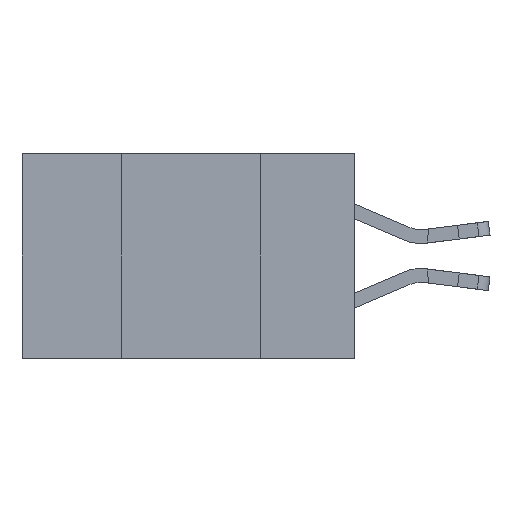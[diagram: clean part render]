
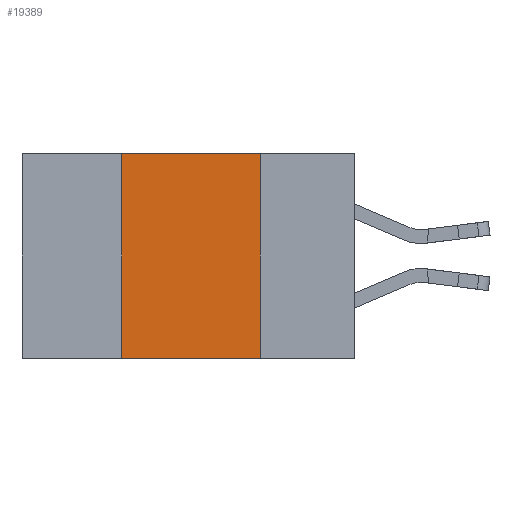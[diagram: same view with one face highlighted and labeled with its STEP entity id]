
A CAD part, left-side view. The second image highlights one B-rep face of the part: STEP entity #19389.
In plain terms, the highlighted planar face has unit normal (-1, 0, 0).
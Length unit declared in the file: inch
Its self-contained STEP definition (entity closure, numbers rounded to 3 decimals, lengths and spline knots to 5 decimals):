
#376 = VERTEX_POINT ( 'NONE', #18928 ) ;
#481 = DIRECTION ( 'NONE',  ( 0., 0., -1. ) ) ;
#744 = DIRECTION ( 'NONE',  ( 1., 0., 0. ) ) ;
#2223 = CARTESIAN_POINT ( 'NONE',  ( 0., 0.6, -0.37 ) ) ;
#2421 = VECTOR ( 'NONE', #27129, 39.37008 ) ;
#3579 = FACE_OUTER_BOUND ( 'NONE', #21615, .T. ) ;
#3930 = EDGE_CURVE ( 'NONE', #25230, #376, #16980, .T. ) ;
#8381 = EDGE_CURVE ( 'NONE', #25230, #9437, #23969, .T. ) ;
#9437 = VERTEX_POINT ( 'NONE', #22293 ) ;
#9518 = CARTESIAN_POINT ( 'NONE',  ( 0., 0.6, 0. ) ) ;
#10086 = VECTOR ( 'NONE', #481, 39.37008 ) ;
#10297 = EDGE_CURVE ( 'NONE', #9437, #14300, #23218, .T. ) ;
#10596 = VECTOR ( 'NONE', #22713, 39.37008 ) ;
#11652 = PLANE ( 'NONE',  #14975 ) ;
#12398 = CARTESIAN_POINT ( 'NONE',  ( 0., 0.42, 0. ) ) ;
#13794 = CARTESIAN_POINT ( 'NONE',  ( 0., 0.17, 0. ) ) ;
#14270 = EDGE_CURVE ( 'NONE', #14300, #376, #21429, .T. ) ;
#14300 = VERTEX_POINT ( 'NONE', #13794 ) ;
#14547 = CARTESIAN_POINT ( 'NONE',  ( 0., 0.42, -0.37 ) ) ;
#14975 = AXIS2_PLACEMENT_3D ( 'NONE', #9518, #744, #16074 ) ;
#16074 = DIRECTION ( 'NONE',  ( 0., 0., -1. ) ) ;
#16980 = LINE ( 'NONE', #2223, #21857 ) ;
#17047 = DIRECTION ( 'NONE',  ( 0., -1., 0. ) ) ;
#17156 = ORIENTED_EDGE ( 'NONE', *, *, #8381, .F. ) ;
#17933 = CARTESIAN_POINT ( 'NONE',  ( 0., 0.17, 0. ) ) ;
#18458 = ORIENTED_EDGE ( 'NONE', *, *, #3930, .T. ) ;
#18504 = CARTESIAN_POINT ( 'NONE',  ( 0., 0.6, 0. ) ) ;
#18928 = CARTESIAN_POINT ( 'NONE',  ( 0., 0.17, -0.37 ) ) ;
#19389 = ADVANCED_FACE ( 'NONE', ( #3579 ), #11652, .F. ) ;
#21429 = LINE ( 'NONE', #17933, #10086 ) ;
#21615 = EDGE_LOOP ( 'NONE', ( #27305, #23686, #17156, #18458 ) ) ;
#21857 = VECTOR ( 'NONE', #17047, 39.37008 ) ;
#22293 = CARTESIAN_POINT ( 'NONE',  ( 0., 0.42, 0. ) ) ;
#22713 = DIRECTION ( 'NONE',  ( 0., -1., 0. ) ) ;
#23218 = LINE ( 'NONE', #18504, #10596 ) ;
#23686 = ORIENTED_EDGE ( 'NONE', *, *, #10297, .F. ) ;
#23969 = LINE ( 'NONE', #12398, #2421 ) ;
#25230 = VERTEX_POINT ( 'NONE', #14547 ) ;
#27129 = DIRECTION ( 'NONE',  ( 0., 0., 1. ) ) ;
#27305 = ORIENTED_EDGE ( 'NONE', *, *, #14270, .F. ) ;
